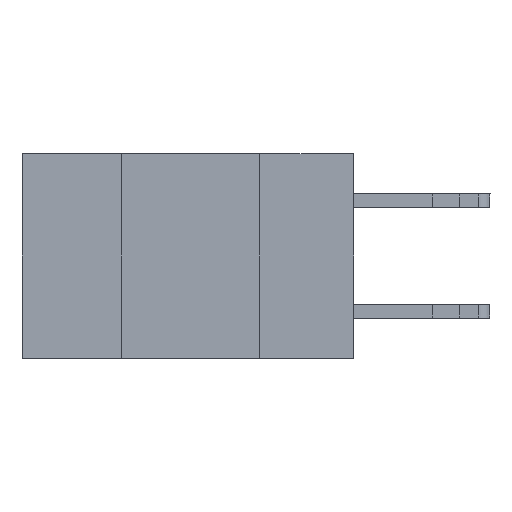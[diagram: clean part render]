
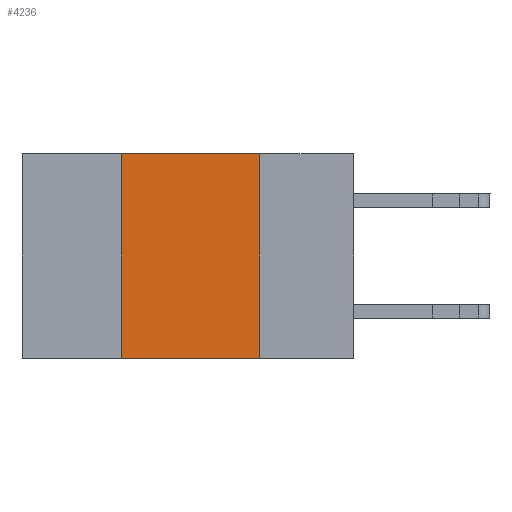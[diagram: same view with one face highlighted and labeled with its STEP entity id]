
A CAD part, left-side view. The second image highlights one B-rep face of the part: STEP entity #4236.
In plain terms, the highlighted planar face has unit normal (-1, 0, 0).
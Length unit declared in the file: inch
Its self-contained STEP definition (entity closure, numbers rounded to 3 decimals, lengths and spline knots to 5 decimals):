
#107 = VECTOR ( 'NONE', #20090, 39.37008 ) ;
#618 = DIRECTION ( 'NONE',  ( 0., 0., -1. ) ) ;
#2060 = VECTOR ( 'NONE', #21967, 39.37008 ) ;
#2440 = EDGE_CURVE ( 'NONE', #19698, #17228, #21577, .T. ) ;
#3245 = CARTESIAN_POINT ( 'NONE',  ( 0., 0.6, 0. ) ) ;
#3469 = LINE ( 'NONE', #22725, #107 ) ;
#4236 = ADVANCED_FACE ( 'NONE', ( #34282 ), #8468, .F. ) ;
#5726 = VECTOR ( 'NONE', #9431, 39.37008 ) ;
#6410 = CARTESIAN_POINT ( 'NONE',  ( 0., 0.42, 0. ) ) ;
#8468 = PLANE ( 'NONE',  #13797 ) ;
#9022 = DIRECTION ( 'NONE',  ( 0., 0., -1. ) ) ;
#9299 = VERTEX_POINT ( 'NONE', #9542 ) ;
#9431 = DIRECTION ( 'NONE',  ( 0., -1., 0. ) ) ;
#9542 = CARTESIAN_POINT ( 'NONE',  ( 0., 0.17, -0.37 ) ) ;
#9892 = CARTESIAN_POINT ( 'NONE',  ( 0., 0.6, -0.37 ) ) ;
#10766 = LINE ( 'NONE', #9892, #5726 ) ;
#11519 = EDGE_CURVE ( 'NONE', #17228, #9299, #30223, .T. ) ;
#11882 = ORIENTED_EDGE ( 'NONE', *, *, #2440, .F. ) ;
#12148 = ORIENTED_EDGE ( 'NONE', *, *, #31324, .T. ) ;
#12580 = ORIENTED_EDGE ( 'NONE', *, *, #32624, .F. ) ;
#13797 = AXIS2_PLACEMENT_3D ( 'NONE', #3245, #24607, #618 ) ;
#16675 = CARTESIAN_POINT ( 'NONE',  ( 0., 0.6, 0. ) ) ;
#17228 = VERTEX_POINT ( 'NONE', #23345 ) ;
#19698 = VERTEX_POINT ( 'NONE', #6410 ) ;
#19914 = VERTEX_POINT ( 'NONE', #26150 ) ;
#20090 = DIRECTION ( 'NONE',  ( 0., 0., 1. ) ) ;
#21577 = LINE ( 'NONE', #16675, #2060 ) ;
#21967 = DIRECTION ( 'NONE',  ( 0., -1., 0. ) ) ;
#22232 = CARTESIAN_POINT ( 'NONE',  ( 0., 0.17, 0. ) ) ;
#22725 = CARTESIAN_POINT ( 'NONE',  ( 0., 0.42, 0. ) ) ;
#23345 = CARTESIAN_POINT ( 'NONE',  ( 0., 0.17, 0. ) ) ;
#24607 = DIRECTION ( 'NONE',  ( 1., 0., 0. ) ) ;
#25443 = EDGE_LOOP ( 'NONE', ( #27573, #11882, #12580, #12148 ) ) ;
#26150 = CARTESIAN_POINT ( 'NONE',  ( 0., 0.42, -0.37 ) ) ;
#26918 = VECTOR ( 'NONE', #9022, 39.37008 ) ;
#27573 = ORIENTED_EDGE ( 'NONE', *, *, #11519, .F. ) ;
#30223 = LINE ( 'NONE', #22232, #26918 ) ;
#31324 = EDGE_CURVE ( 'NONE', #19914, #9299, #10766, .T. ) ;
#32624 = EDGE_CURVE ( 'NONE', #19914, #19698, #3469, .T. ) ;
#34282 = FACE_OUTER_BOUND ( 'NONE', #25443, .T. ) ;
